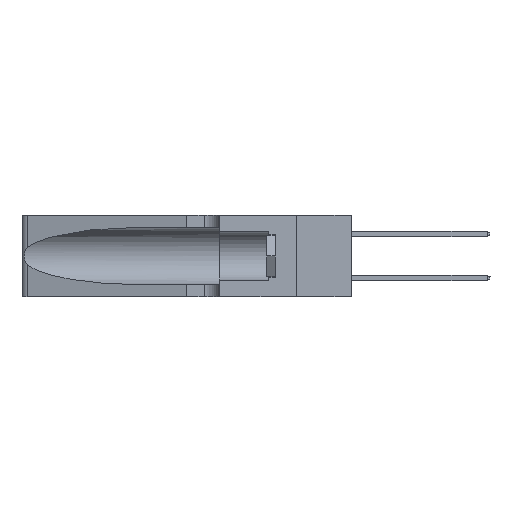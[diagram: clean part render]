
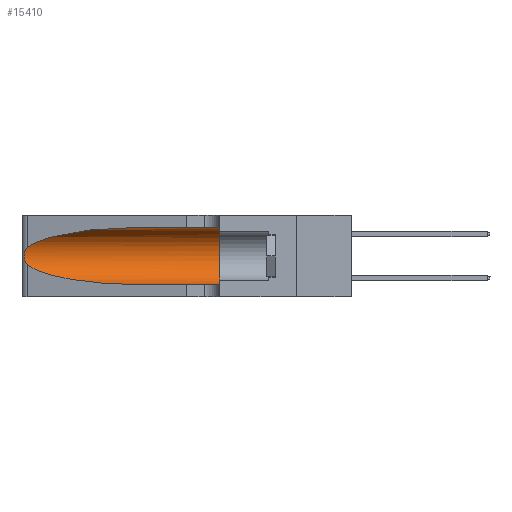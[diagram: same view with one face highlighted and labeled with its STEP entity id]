
A CAD part, left-side view. The second image highlights one B-rep face of the part: STEP entity #15410.
In plain terms, the highlighted cylindrical face has radius 3.308 mm (diameter 6.617 mm), a partial arc.
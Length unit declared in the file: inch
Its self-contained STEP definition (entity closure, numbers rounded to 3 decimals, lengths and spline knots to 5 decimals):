
#3456 = CARTESIAN_POINT ( 'NONE',  ( 0.25789, 1.23486, 0.15765 ) ) ;
#5255 = CARTESIAN_POINT ( 'NONE',  ( 0.1305, 1.61858, 0.31525 ) ) ;
#6359 = FACE_OUTER_BOUND ( 'NONE', #25493, .T. ) ;
#6422 = ORIENTED_EDGE ( 'NONE', *, *, #29535, .T. ) ;
#7066 = CARTESIAN_POINT ( 'NONE',  ( 0.25487, 1.22718, 0.22369 ) ) ;
#7182 = CARTESIAN_POINT ( 'NONE',  ( 0.25555, 1.22993, 0.14849 ) ) ;
#7195 = VERTEX_POINT ( 'NONE', #25067 ) ;
#9177 = ORIENTED_EDGE ( 'NONE', *, *, #34327, .F. ) ;
#9615 = DIRECTION ( 'NONE',  ( 0., 1., 0. ) ) ;
#10502 = CARTESIAN_POINT ( 'NONE',  ( 0.1305, 0.72297, 0.05475 ) ) ;
#10861 = CARTESIAN_POINT ( 'NONE',  ( 0.2373, 1.15595, 0.28018 ) ) ;
#12169 = DIRECTION ( 'NONE',  ( 0., 0., -1. ) ) ;
#13108 = DIRECTION ( 'NONE',  ( 0., -1., 0. ) ) ;
#13114 = VERTEX_POINT ( 'NONE', #25766 ) ;
#13195 = CARTESIAN_POINT ( 'NONE',  ( 0.25787, 1.23484, 0.2124 ) ) ;
#14236 = CARTESIAN_POINT ( 'NONE',  ( 0.1305, 0.72297, 0.31525 ) ) ;
#14465 = VERTEX_POINT ( 'NONE', #10502 ) ;
#15272 = VERTEX_POINT ( 'NONE', #42760 ) ;
#15410 = ADVANCED_FACE ( 'NONE', ( #6359 ), #32936, .F. ) ;
#15904 = CARTESIAN_POINT ( 'NONE',  ( 0.2373, 1.15595, 0.08982 ) ) ;
#15981 = AXIS2_PLACEMENT_3D ( 'NONE', #16324, #9615, #33461 ) ;
#16324 = CARTESIAN_POINT ( 'NONE',  ( 0.1305, 0.35, 0.185 ) ) ;
#16732 = CARTESIAN_POINT ( 'NONE',  ( 0.1305, 1.61858, 0.05475 ) ) ;
#17801 = CARTESIAN_POINT ( 'NONE',  ( 0.25487, 1.22718, 0.14631 ) ) ;
#19235 = CARTESIAN_POINT ( 'NONE',  ( 0.25487, 1.22718, 0.14631 ) ) ;
#19856 = CARTESIAN_POINT ( 'NONE',  ( 0.25487, 1.22718, 0.22369 ) ) ;
#20040 = EDGE_CURVE ( 'NONE', #14465, #28147, #21966, .T. ) ;
#20873 = CARTESIAN_POINT ( 'NONE',  ( 0.25639, 1.23186, 0.15144 ) ) ;
#21704 = VECTOR ( 'NONE', #39519, 39.37008 ) ;
#21966 = LINE ( 'NONE', #16732, #23085 ) ;
#22763 = EDGE_CURVE ( 'NONE', #15272, #7195, #44869, .T. ) ;
#23085 = VECTOR ( 'NONE', #13108, 39.37008 ) ;
#23147 = CARTESIAN_POINT ( 'NONE',  ( 0.18966, 0.96281, 0.05475 ) ) ;
#23748 = CARTESIAN_POINT ( 'NONE',  ( 0.1305, 0.35, 0.31525 ) ) ;
#23983 = CARTESIAN_POINT ( 'NONE',  ( 0.1305, 0.35, 0.05475 ) ) ;
#24358 = CARTESIAN_POINT ( 'NONE',  ( 0.25856, 1.23593, 0.16098 ) ) ;
#25067 = CARTESIAN_POINT ( 'NONE',  ( 0.25487, 1.22718, 0.14631 ) ) ;
#25493 = EDGE_LOOP ( 'NONE', ( #28725, #44175, #6422, #35637, #9177, #42944 ) ) ;
#25561 = CIRCLE ( 'NONE', #15981, 0.13025 ) ;
#25667 = AXIS2_PLACEMENT_3D ( 'NONE', #43617, #44057, #12169 ) ;
#25766 = CARTESIAN_POINT ( 'NONE',  ( 0.1305, 0.72297, 0.31525 ) ) ;
#25831 = EDGE_CURVE ( 'NONE', #13114, #15272, #33457, .T. ) ;
#28147 = VERTEX_POINT ( 'NONE', #23983 ) ;
#28725 = ORIENTED_EDGE ( 'NONE', *, *, #25831, .T. ) ;
#29535 = EDGE_CURVE ( 'NONE', #7195, #14465, #42080, .T. ) ;
#30000 = VERTEX_POINT ( 'NONE', #23748 ) ;
#32936 = CYLINDRICAL_SURFACE ( 'NONE', #25667, 0.13025 ) ;
#33457 =( BOUNDED_CURVE ( )  B_SPLINE_CURVE ( 3, ( #14236, #38347, #10861, #7066 ),
 .UNSPECIFIED., .F., .F. ) 
 B_SPLINE_CURVE_WITH_KNOTS ( ( 4, 4 ),
 ( 1.5708, 2.84003 ),
 .UNSPECIFIED. ) 
 CURVE ( )  GEOMETRIC_REPRESENTATION_ITEM ( )  RATIONAL_B_SPLINE_CURVE ( ( 1., 0.87, 0.87, 1. ) ) 
 REPRESENTATION_ITEM ( '' )  );
#33461 = DIRECTION ( 'NONE',  ( 0., 0., 1. ) ) ;
#34098 = CARTESIAN_POINT ( 'NONE',  ( 0.26075, 1.23896, 0.19203 ) ) ;
#34327 = EDGE_CURVE ( 'NONE', #30000, #28147, #25561, .T. ) ;
#35637 = ORIENTED_EDGE ( 'NONE', *, *, #20040, .T. ) ;
#37430 = CARTESIAN_POINT ( 'NONE',  ( 0.25854, 1.2359, 0.20912 ) ) ;
#37584 = CARTESIAN_POINT ( 'NONE',  ( 0.26075, 1.23896, 0.178 ) ) ;
#38347 = CARTESIAN_POINT ( 'NONE',  ( 0.18966, 0.96281, 0.31525 ) ) ;
#39084 = LINE ( 'NONE', #5255, #21704 ) ;
#39519 = DIRECTION ( 'NONE',  ( 0., -1., 0. ) ) ;
#40179 = CARTESIAN_POINT ( 'NONE',  ( 0.1305, 0.72297, 0.05475 ) ) ;
#40944 = CARTESIAN_POINT ( 'NONE',  ( 0.26018, 1.23835, 0.19895 ) ) ;
#41097 = CARTESIAN_POINT ( 'NONE',  ( 0.26017, 1.23833, 0.17102 ) ) ;
#42080 =( BOUNDED_CURVE ( )  B_SPLINE_CURVE ( 3, ( #19235, #15904, #23147, #40179 ),
 .UNSPECIFIED., .F., .F. ) 
 B_SPLINE_CURVE_WITH_KNOTS ( ( 4, 4 ),
 ( 3.44316, 4.71239 ),
 .UNSPECIFIED. ) 
 CURVE ( )  GEOMETRIC_REPRESENTATION_ITEM ( )  RATIONAL_B_SPLINE_CURVE ( ( 1., 0.87, 0.87, 1. ) ) 
 REPRESENTATION_ITEM ( '' )  );
#42760 = CARTESIAN_POINT ( 'NONE',  ( 0.25487, 1.22718, 0.22369 ) ) ;
#42762 = EDGE_CURVE ( 'NONE', #13114, #30000, #39084, .T. ) ;
#42944 = ORIENTED_EDGE ( 'NONE', *, *, #42762, .F. ) ;
#43560 = CARTESIAN_POINT ( 'NONE',  ( 0.25639, 1.23184, 0.21858 ) ) ;
#43617 = CARTESIAN_POINT ( 'NONE',  ( 0.1305, 1.61858, 0.185 ) ) ;
#44057 = DIRECTION ( 'NONE',  ( 0., -1., 0. ) ) ;
#44143 = CARTESIAN_POINT ( 'NONE',  ( 0.25555, 1.22994, 0.2215 ) ) ;
#44175 = ORIENTED_EDGE ( 'NONE', *, *, #22763, .T. ) ;
#44869 = B_SPLINE_CURVE_WITH_KNOTS ( 'NONE', 3,
 ( #19856, #44143, #43560, #13195, #37430, #40944, #34098, #37584, #41097, #24358, #3456, #20873, #7182, #17801 ),
 .UNSPECIFIED., .F., .F.,
 ( 4, 2, 2, 2, 2, 2, 4 ),
 ( 0., 0.00027, 0.00053, 0.00107, 0.0016, 0.00187, 0.00214 ),
 .UNSPECIFIED. ) ;
